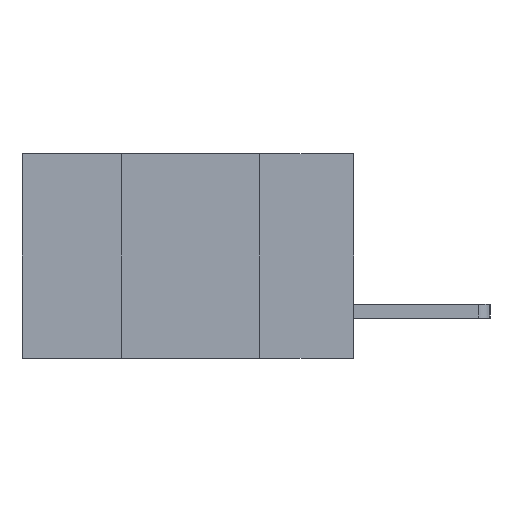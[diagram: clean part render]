
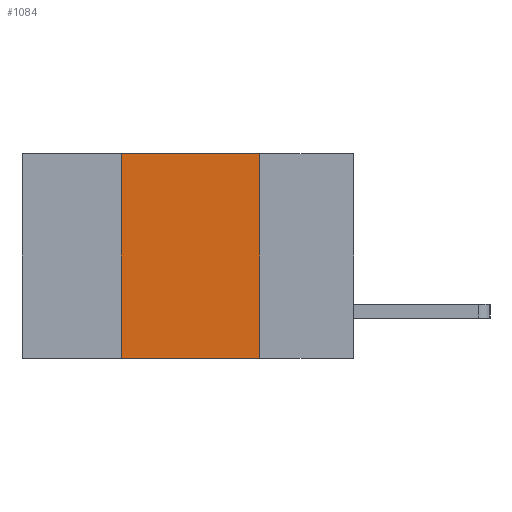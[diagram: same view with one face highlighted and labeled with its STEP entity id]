
A CAD part, left-side view. The second image highlights one B-rep face of the part: STEP entity #1084.
In plain terms, the highlighted planar face has unit normal (-1, 0, 0).
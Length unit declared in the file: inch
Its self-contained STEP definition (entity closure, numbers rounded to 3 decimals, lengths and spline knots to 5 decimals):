
#303 = LINE ( 'NONE', #8394, #5673 ) ;
#593 = VECTOR ( 'NONE', #6731, 39.37008 ) ;
#689 = EDGE_CURVE ( 'NONE', #9594, #1926, #303, .T. ) ;
#1084 = ADVANCED_FACE ( 'NONE', ( #6738 ), #11784, .F. ) ;
#1926 = VERTEX_POINT ( 'NONE', #9323 ) ;
#2250 = LINE ( 'NONE', #6284, #12321 ) ;
#2770 = CARTESIAN_POINT ( 'NONE',  ( 0., 0.6, 0. ) ) ;
#2839 = LINE ( 'NONE', #6873, #593 ) ;
#3325 = DIRECTION ( 'NONE',  ( 0., -1., 0. ) ) ;
#3662 = ORIENTED_EDGE ( 'NONE', *, *, #689, .T. ) ;
#4518 = CARTESIAN_POINT ( 'NONE',  ( 0., 0.17, 0. ) ) ;
#5306 = LINE ( 'NONE', #8441, #8795 ) ;
#5307 = EDGE_CURVE ( 'NONE', #9594, #12402, #2250, .T. ) ;
#5673 = VECTOR ( 'NONE', #12429, 39.37008 ) ;
#5902 = EDGE_LOOP ( 'NONE', ( #11064, #12170, #7617, #3662 ) ) ;
#6284 = CARTESIAN_POINT ( 'NONE',  ( 0., 0.42, 0. ) ) ;
#6648 = CARTESIAN_POINT ( 'NONE',  ( 0., 0.42, -0.37 ) ) ;
#6731 = DIRECTION ( 'NONE',  ( 0., 0., -1. ) ) ;
#6738 = FACE_OUTER_BOUND ( 'NONE', #5902, .T. ) ;
#6860 = VERTEX_POINT ( 'NONE', #4518 ) ;
#6873 = CARTESIAN_POINT ( 'NONE',  ( 0., 0.17, 0. ) ) ;
#7393 = AXIS2_PLACEMENT_3D ( 'NONE', #2770, #10852, #10715 ) ;
#7617 = ORIENTED_EDGE ( 'NONE', *, *, #5307, .F. ) ;
#8394 = CARTESIAN_POINT ( 'NONE',  ( 0., 0.6, -0.37 ) ) ;
#8441 = CARTESIAN_POINT ( 'NONE',  ( 0., 0.6, 0. ) ) ;
#8795 = VECTOR ( 'NONE', #3325, 39.37008 ) ;
#9282 = EDGE_CURVE ( 'NONE', #12402, #6860, #5306, .T. ) ;
#9323 = CARTESIAN_POINT ( 'NONE',  ( 0., 0.17, -0.37 ) ) ;
#9594 = VERTEX_POINT ( 'NONE', #6648 ) ;
#10460 = DIRECTION ( 'NONE',  ( 0., 0., 1. ) ) ;
#10715 = DIRECTION ( 'NONE',  ( 0., 0., -1. ) ) ;
#10852 = DIRECTION ( 'NONE',  ( 1., 0., 0. ) ) ;
#11064 = ORIENTED_EDGE ( 'NONE', *, *, #12230, .F. ) ;
#11250 = CARTESIAN_POINT ( 'NONE',  ( 0., 0.42, 0. ) ) ;
#11784 = PLANE ( 'NONE',  #7393 ) ;
#12170 = ORIENTED_EDGE ( 'NONE', *, *, #9282, .F. ) ;
#12230 = EDGE_CURVE ( 'NONE', #6860, #1926, #2839, .T. ) ;
#12321 = VECTOR ( 'NONE', #10460, 39.37008 ) ;
#12402 = VERTEX_POINT ( 'NONE', #11250 ) ;
#12429 = DIRECTION ( 'NONE',  ( 0., -1., 0. ) ) ;
